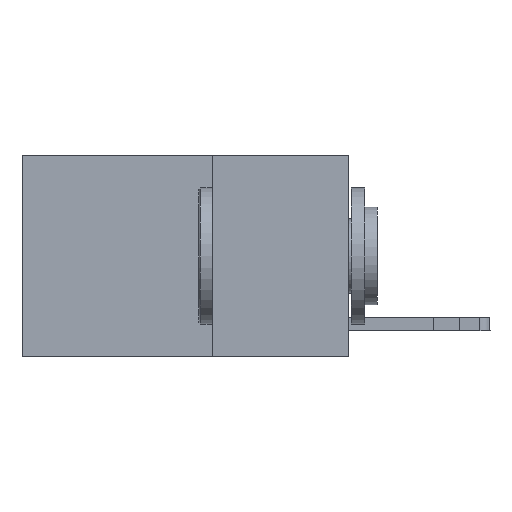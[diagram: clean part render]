
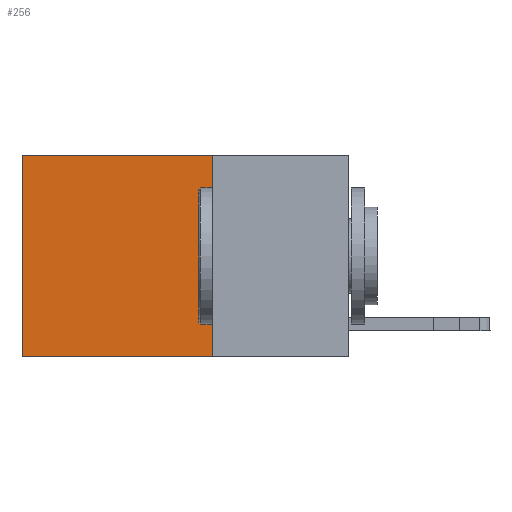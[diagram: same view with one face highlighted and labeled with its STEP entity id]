
A CAD part, left-side view. The second image highlights one B-rep face of the part: STEP entity #256.
In plain terms, the highlighted planar face has unit normal (-1, 0, 0).
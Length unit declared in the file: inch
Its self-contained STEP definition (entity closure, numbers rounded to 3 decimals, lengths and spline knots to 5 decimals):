
#35 = EDGE_CURVE ( 'NONE', #2941, #376, #377, .T. ) ;
#256 = ADVANCED_FACE ( 'NONE', ( #2631 ), #3766, .F. ) ;
#319 = CARTESIAN_POINT ( 'NONE',  ( 0.2625, 0.6, 0. ) ) ;
#368 = ORIENTED_EDGE ( 'NONE', *, *, #35, .T. ) ;
#376 = VERTEX_POINT ( 'NONE', #10791 ) ;
#377 = LINE ( 'NONE', #6336, #11588 ) ;
#890 = VERTEX_POINT ( 'NONE', #7330 ) ;
#1925 = EDGE_CURVE ( 'NONE', #11964, #376, #10139, .T. ) ;
#2387 = CARTESIAN_POINT ( 'NONE',  ( 0.2625, 0.25, 0. ) ) ;
#2514 = LINE ( 'NONE', #2387, #11556 ) ;
#2631 = FACE_OUTER_BOUND ( 'NONE', #2718, .T. ) ;
#2718 = EDGE_LOOP ( 'NONE', ( #368, #3007, #7493, #11783 ) ) ;
#2803 = AXIS2_PLACEMENT_3D ( 'NONE', #5803, #10612, #6598 ) ;
#2941 = VERTEX_POINT ( 'NONE', #319 ) ;
#3007 = ORIENTED_EDGE ( 'NONE', *, *, #1925, .F. ) ;
#3766 = PLANE ( 'NONE',  #2803 ) ;
#3777 = EDGE_CURVE ( 'NONE', #890, #2941, #2514, .T. ) ;
#4800 = LINE ( 'NONE', #8064, #9629 ) ;
#5110 = CARTESIAN_POINT ( 'NONE',  ( 0.2625, 0.25, -0.37 ) ) ;
#5803 = CARTESIAN_POINT ( 'NONE',  ( 0.2625, 0.25, 0. ) ) ;
#6336 = CARTESIAN_POINT ( 'NONE',  ( 0.2625, 0.6, 0. ) ) ;
#6598 = DIRECTION ( 'NONE',  ( 0., 0., -1. ) ) ;
#7330 = CARTESIAN_POINT ( 'NONE',  ( 0.2625, 0.25, 0. ) ) ;
#7493 = ORIENTED_EDGE ( 'NONE', *, *, #12612, .F. ) ;
#7583 = DIRECTION ( 'NONE',  ( 0., 1., 0. ) ) ;
#8064 = CARTESIAN_POINT ( 'NONE',  ( 0.2625, 0.25, 0. ) ) ;
#8481 = DIRECTION ( 'NONE',  ( 0., 0., -1. ) ) ;
#9006 = CARTESIAN_POINT ( 'NONE',  ( 0.2625, 0.25, -0.37 ) ) ;
#9629 = VECTOR ( 'NONE', #10979, 39.37008 ) ;
#9993 = DIRECTION ( 'NONE',  ( 0., 1., 0. ) ) ;
#10139 = LINE ( 'NONE', #5110, #11649 ) ;
#10612 = DIRECTION ( 'NONE',  ( 1., 0., 0. ) ) ;
#10791 = CARTESIAN_POINT ( 'NONE',  ( 0.2625, 0.6, -0.37 ) ) ;
#10979 = DIRECTION ( 'NONE',  ( 0., 0., -1. ) ) ;
#11556 = VECTOR ( 'NONE', #7583, 39.37008 ) ;
#11588 = VECTOR ( 'NONE', #8481, 39.37008 ) ;
#11649 = VECTOR ( 'NONE', #9993, 39.37008 ) ;
#11783 = ORIENTED_EDGE ( 'NONE', *, *, #3777, .T. ) ;
#11964 = VERTEX_POINT ( 'NONE', #9006 ) ;
#12612 = EDGE_CURVE ( 'NONE', #890, #11964, #4800, .T. ) ;
